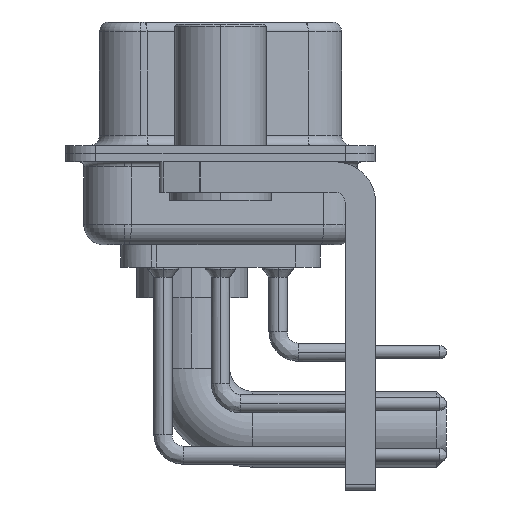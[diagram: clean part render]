
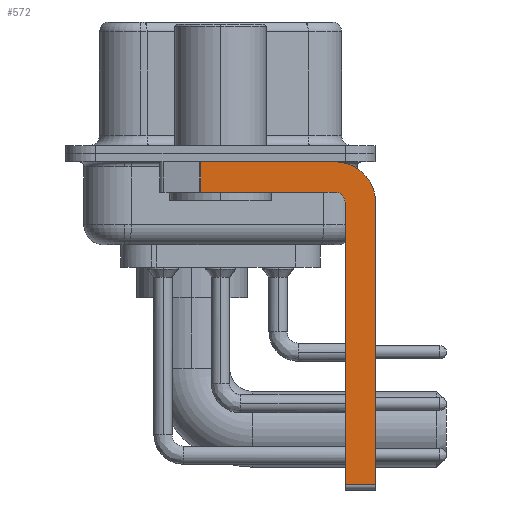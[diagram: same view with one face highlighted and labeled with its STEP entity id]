
A CAD part, left-side view. The second image highlights one B-rep face of the part: STEP entity #572.
In plain terms, the highlighted planar face has unit normal (-1, 0, 0).
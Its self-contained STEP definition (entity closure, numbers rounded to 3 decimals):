
#572 = ADVANCED_FACE ( 'NONE', ( #31339 ), #28312, .F. ) ;
#1292 = DIRECTION ( 'NONE',  ( 0., 0., -1. ) ) ;
#1750 = VERTEX_POINT ( 'NONE', #5397 ) ;
#2157 = VECTOR ( 'NONE', #25495, 1000. ) ;
#2193 = CARTESIAN_POINT ( 'NONE',  ( -2.9, 0.978, -0.4 ) ) ;
#2442 = AXIS2_PLACEMENT_3D ( 'NONE', #17137, #38968, #19772 ) ;
#3308 = CARTESIAN_POINT ( 'NONE',  ( -2.9, -7.65, -16.35 ) ) ;
#3347 = VECTOR ( 'NONE', #23242, 1000. ) ;
#3557 = VERTEX_POINT ( 'NONE', #30989 ) ;
#4677 = EDGE_CURVE ( 'NONE', #3557, #27710, #7826, .T. ) ;
#5102 = EDGE_CURVE ( 'NONE', #17175, #39399, #18435, .T. ) ;
#5397 = CARTESIAN_POINT ( 'NONE',  ( -2.9, -6.15, -16.35 ) ) ;
#5569 = EDGE_CURVE ( 'NONE', #17175, #31521, #33144, .T. ) ;
#6385 = CARTESIAN_POINT ( 'NONE',  ( -2.9, -5.65, -2.4 ) ) ;
#6740 = CARTESIAN_POINT ( 'NONE',  ( -2.9, -5.65, -1.9 ) ) ;
#7710 = ORIENTED_EDGE ( 'NONE', *, *, #14327, .F. ) ;
#7826 = CIRCLE ( 'NONE', #23920, 0.5 ) ;
#8547 = EDGE_CURVE ( 'NONE', #1750, #14742, #12404, .T. ) ;
#8684 = LINE ( 'NONE', #14326, #9009 ) ;
#9009 = VECTOR ( 'NONE', #23401, 1000. ) ;
#9821 = ORIENTED_EDGE ( 'NONE', *, *, #14190, .F. ) ;
#10804 = CIRCLE ( 'NONE', #2442, 2. ) ;
#11561 = CARTESIAN_POINT ( 'NONE',  ( -2.9, -5.65, -1.9 ) ) ;
#11806 = CARTESIAN_POINT ( 'NONE',  ( -2.9, 3., -0.4 ) ) ;
#12346 = CARTESIAN_POINT ( 'NONE',  ( -2.9, 0.978, -1.9 ) ) ;
#12404 = LINE ( 'NONE', #27924, #2157 ) ;
#13489 = ORIENTED_EDGE ( 'NONE', *, *, #4677, .F. ) ;
#14190 = EDGE_CURVE ( 'NONE', #39399, #27939, #10804, .T. ) ;
#14326 = CARTESIAN_POINT ( 'NONE',  ( -2.9, -7.65, -2.4 ) ) ;
#14327 = EDGE_CURVE ( 'NONE', #1750, #3557, #33087, .T. ) ;
#14742 = VERTEX_POINT ( 'NONE', #3308 ) ;
#15830 = VECTOR ( 'NONE', #36570, 1000. ) ;
#17137 = CARTESIAN_POINT ( 'NONE',  ( -2.9, -5.65, -2.4 ) ) ;
#17175 = VERTEX_POINT ( 'NONE', #2193 ) ;
#17731 = CARTESIAN_POINT ( 'NONE',  ( -2.9, -6.15, -16.6 ) ) ;
#18011 = CARTESIAN_POINT ( 'NONE',  ( -2.9, -7.65, -2.4 ) ) ;
#18435 = LINE ( 'NONE', #11806, #24204 ) ;
#19772 = DIRECTION ( 'NONE',  ( 0., 0., -1. ) ) ;
#22529 = CARTESIAN_POINT ( 'NONE',  ( -2.9, 0.978, -1.9 ) ) ;
#22915 = EDGE_LOOP ( 'NONE', ( #29246, #28369, #35532, #13489, #7710, #28413, #39278, #9821 ) ) ;
#23242 = DIRECTION ( 'NONE',  ( 0., 1., 0. ) ) ;
#23401 = DIRECTION ( 'NONE',  ( 0., 0., -1. ) ) ;
#23920 = AXIS2_PLACEMENT_3D ( 'NONE', #6385, #23940, #39913 ) ;
#23940 = DIRECTION ( 'NONE',  ( -1., 0., 0. ) ) ;
#24094 = DIRECTION ( 'NONE',  ( 0., -1., 0. ) ) ;
#24204 = VECTOR ( 'NONE', #24094, 1000. ) ;
#25495 = DIRECTION ( 'NONE',  ( 0., -1., 0. ) ) ;
#25627 = VECTOR ( 'NONE', #39372, 1000. ) ;
#26076 = LINE ( 'NONE', #11561, #3347 ) ;
#26315 = EDGE_CURVE ( 'NONE', #27710, #31521, #26076, .T. ) ;
#26948 = AXIS2_PLACEMENT_3D ( 'NONE', #38415, #34781, #1292 ) ;
#27710 = VERTEX_POINT ( 'NONE', #6740 ) ;
#27924 = CARTESIAN_POINT ( 'NONE',  ( -2.9, -5.65, -16.35 ) ) ;
#27939 = VERTEX_POINT ( 'NONE', #18011 ) ;
#28312 = PLANE ( 'NONE',  #26948 ) ;
#28369 = ORIENTED_EDGE ( 'NONE', *, *, #5569, .T. ) ;
#28413 = ORIENTED_EDGE ( 'NONE', *, *, #8547, .T. ) ;
#29246 = ORIENTED_EDGE ( 'NONE', *, *, #5102, .F. ) ;
#29420 = EDGE_CURVE ( 'NONE', #27939, #14742, #8684, .T. ) ;
#30989 = CARTESIAN_POINT ( 'NONE',  ( -2.9, -6.15, -2.4 ) ) ;
#31339 = FACE_OUTER_BOUND ( 'NONE', #22915, .T. ) ;
#31521 = VERTEX_POINT ( 'NONE', #22529 ) ;
#33087 = LINE ( 'NONE', #17731, #25627 ) ;
#33144 = LINE ( 'NONE', #12346, #15830 ) ;
#34781 = DIRECTION ( 'NONE',  ( 1., 0., 0. ) ) ;
#35532 = ORIENTED_EDGE ( 'NONE', *, *, #26315, .F. ) ;
#36570 = DIRECTION ( 'NONE',  ( 0., 0., -1. ) ) ;
#38347 = CARTESIAN_POINT ( 'NONE',  ( -2.9, -5.65, -0.4 ) ) ;
#38415 = CARTESIAN_POINT ( 'NONE',  ( -2.9, -5.65, -2.4 ) ) ;
#38968 = DIRECTION ( 'NONE',  ( 1., 0., 0. ) ) ;
#39278 = ORIENTED_EDGE ( 'NONE', *, *, #29420, .F. ) ;
#39372 = DIRECTION ( 'NONE',  ( 0., 0., 1. ) ) ;
#39399 = VERTEX_POINT ( 'NONE', #38347 ) ;
#39913 = DIRECTION ( 'NONE',  ( 0., 0., 1. ) ) ;
